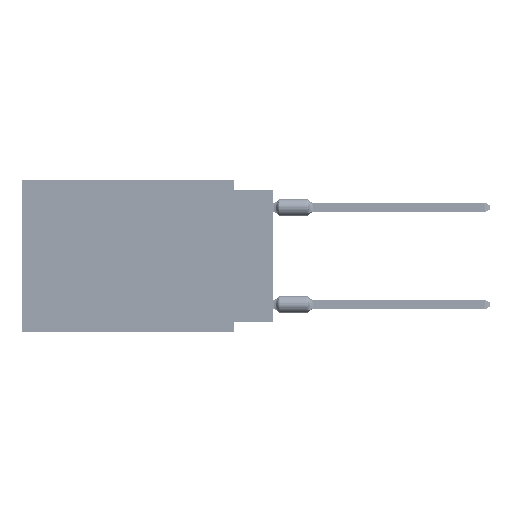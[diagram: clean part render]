
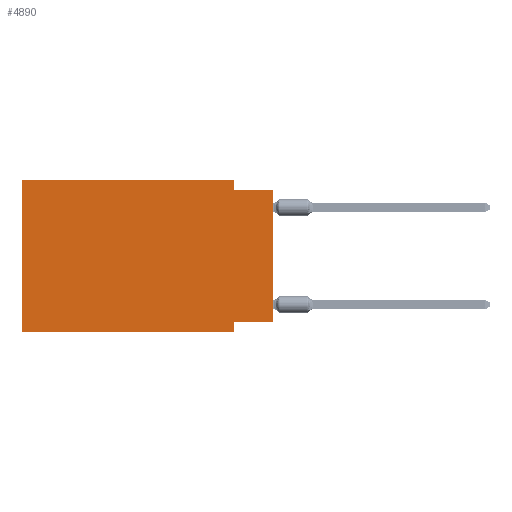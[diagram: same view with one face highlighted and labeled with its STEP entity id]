
A CAD part, left-side view. The second image highlights one B-rep face of the part: STEP entity #4890.
In plain terms, the highlighted planar face has unit normal (-1, 0, 0).
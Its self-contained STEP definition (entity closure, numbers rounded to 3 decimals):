
#1541 = CARTESIAN_POINT ( 'NONE',  ( 0., 2.54, 0. ) ) ;
#3694 = CARTESIAN_POINT ( 'NONE',  ( 0., 0., -9.271 ) ) ;
#4011 = EDGE_CURVE ( 'NONE', #73036, #9170, #19686, .T. ) ;
#4890 = ADVANCED_FACE ( 'NONE', ( #60173 ), #21541, .F. ) ;
#7892 = CARTESIAN_POINT ( 'NONE',  ( 0., 16.383, 0. ) ) ;
#8349 = CARTESIAN_POINT ( 'NONE',  ( 0., 0., 0. ) ) ;
#8694 = DIRECTION ( 'NONE',  ( 0., 0., -1. ) ) ;
#9170 = VERTEX_POINT ( 'NONE', #64772 ) ;
#11286 = CARTESIAN_POINT ( 'NONE',  ( 0., 0., -0.635 ) ) ;
#11437 = EDGE_CURVE ( 'NONE', #49357, #34377, #28725, .T. ) ;
#14482 = CARTESIAN_POINT ( 'NONE',  ( 0., 0., -9.271 ) ) ;
#15237 = CARTESIAN_POINT ( 'NONE',  ( 0., 16.383, 0. ) ) ;
#15415 = LINE ( 'NONE', #1541, #17500 ) ;
#17465 = ORIENTED_EDGE ( 'NONE', *, *, #47326, .F. ) ;
#17500 = VECTOR ( 'NONE', #8694, 1000. ) ;
#19686 = LINE ( 'NONE', #7892, #63370 ) ;
#20045 = VECTOR ( 'NONE', #45591, 1000. ) ;
#21541 = PLANE ( 'NONE',  #25872 ) ;
#24547 = DIRECTION ( 'NONE',  ( 0., -1., 0. ) ) ;
#24682 = DIRECTION ( 'NONE',  ( 0., -1., 0. ) ) ;
#25309 = ORIENTED_EDGE ( 'NONE', *, *, #34892, .F. ) ;
#25872 = AXIS2_PLACEMENT_3D ( 'NONE', #15237, #66484, #36202 ) ;
#25964 = DIRECTION ( 'NONE',  ( 0., 0., 1. ) ) ;
#26088 = EDGE_CURVE ( 'NONE', #26215, #34377, #59582, .T. ) ;
#26215 = VERTEX_POINT ( 'NONE', #3694 ) ;
#27334 = VERTEX_POINT ( 'NONE', #64254 ) ;
#28321 = CARTESIAN_POINT ( 'NONE',  ( 0., 0., -0.635 ) ) ;
#28725 = LINE ( 'NONE', #28321, #60211 ) ;
#29847 = ORIENTED_EDGE ( 'NONE', *, *, #51251, .F. ) ;
#30561 = LINE ( 'NONE', #62496, #65395 ) ;
#33457 = VERTEX_POINT ( 'NONE', #38034 ) ;
#34377 = VERTEX_POINT ( 'NONE', #11286 ) ;
#34863 = ORIENTED_EDGE ( 'NONE', *, *, #71595, .T. ) ;
#34892 = EDGE_CURVE ( 'NONE', #26215, #33457, #39682, .T. ) ;
#36202 = DIRECTION ( 'NONE',  ( 0., 0., -1. ) ) ;
#38021 = VECTOR ( 'NONE', #24547, 1000. ) ;
#38034 = CARTESIAN_POINT ( 'NONE',  ( 0., 2.54, -9.271 ) ) ;
#39682 = LINE ( 'NONE', #14482, #20045 ) ;
#43405 = LINE ( 'NONE', #64364, #57152 ) ;
#43461 = LINE ( 'NONE', #62770, #38021 ) ;
#43780 = ORIENTED_EDGE ( 'NONE', *, *, #60447, .F. ) ;
#45591 = DIRECTION ( 'NONE',  ( 0., 1., 0. ) ) ;
#47326 = EDGE_CURVE ( 'NONE', #9170, #79245, #30561, .T. ) ;
#48811 = ORIENTED_EDGE ( 'NONE', *, *, #11437, .F. ) ;
#49258 = EDGE_LOOP ( 'NONE', ( #49674, #48811, #43780, #17465, #49903, #34863, #29847, #25309 ) ) ;
#49357 = VERTEX_POINT ( 'NONE', #58756 ) ;
#49674 = ORIENTED_EDGE ( 'NONE', *, *, #26088, .T. ) ;
#49903 = ORIENTED_EDGE ( 'NONE', *, *, #4011, .F. ) ;
#51251 = EDGE_CURVE ( 'NONE', #33457, #27334, #43405, .T. ) ;
#57152 = VECTOR ( 'NONE', #63544, 1000. ) ;
#58756 = CARTESIAN_POINT ( 'NONE',  ( 0., 2.54, -0.635 ) ) ;
#59582 = LINE ( 'NONE', #8349, #67406 ) ;
#60173 = FACE_OUTER_BOUND ( 'NONE', #49258, .T. ) ;
#60211 = VECTOR ( 'NONE', #61894, 1000. ) ;
#60447 = EDGE_CURVE ( 'NONE', #79245, #49357, #15415, .T. ) ;
#61894 = DIRECTION ( 'NONE',  ( 0., -1., 0. ) ) ;
#62496 = CARTESIAN_POINT ( 'NONE',  ( 0., 16.383, 0. ) ) ;
#62770 = CARTESIAN_POINT ( 'NONE',  ( 0., 16.383, -9.906 ) ) ;
#63370 = VECTOR ( 'NONE', #25964, 1000. ) ;
#63544 = DIRECTION ( 'NONE',  ( 0., 0., -1. ) ) ;
#64254 = CARTESIAN_POINT ( 'NONE',  ( 0., 2.54, -9.906 ) ) ;
#64364 = CARTESIAN_POINT ( 'NONE',  ( 0., 2.54, -9.906 ) ) ;
#64772 = CARTESIAN_POINT ( 'NONE',  ( 0., 16.383, 0. ) ) ;
#65395 = VECTOR ( 'NONE', #24682, 1000. ) ;
#65462 = DIRECTION ( 'NONE',  ( 0., 0., 1. ) ) ;
#66484 = DIRECTION ( 'NONE',  ( 1., 0., 0. ) ) ;
#67406 = VECTOR ( 'NONE', #65462, 1000. ) ;
#71595 = EDGE_CURVE ( 'NONE', #73036, #27334, #43461, .T. ) ;
#72445 = CARTESIAN_POINT ( 'NONE',  ( 0., 16.383, -9.906 ) ) ;
#73036 = VERTEX_POINT ( 'NONE', #72445 ) ;
#76297 = CARTESIAN_POINT ( 'NONE',  ( 0., 2.54, 0. ) ) ;
#79245 = VERTEX_POINT ( 'NONE', #76297 ) ;
